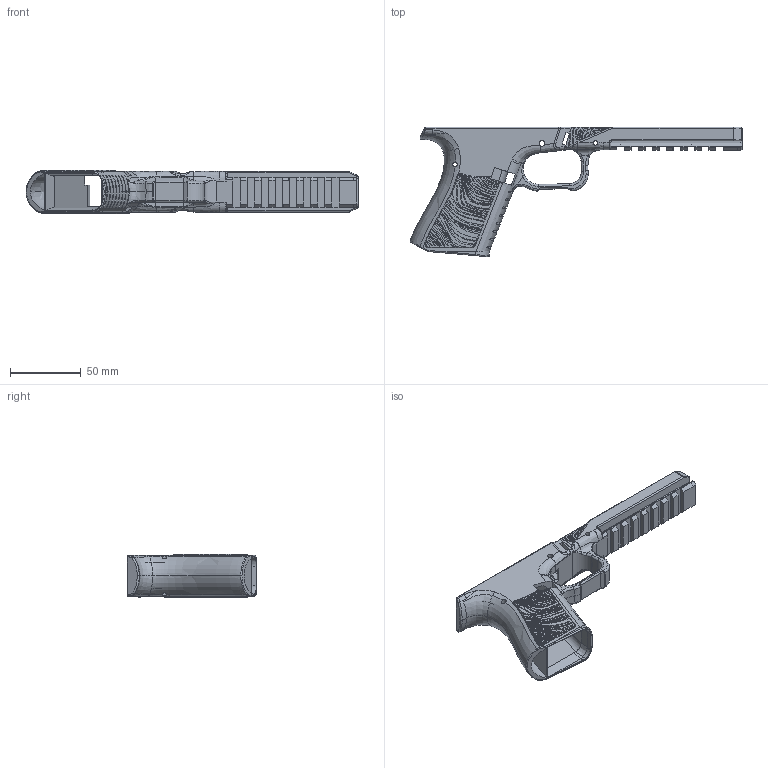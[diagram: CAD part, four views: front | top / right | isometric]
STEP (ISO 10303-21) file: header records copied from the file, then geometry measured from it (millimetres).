
FILE_DESCRIPTION(/* description */ (''),/* implementation_level */ '2;1');
FILE_NAME(/* name */ 'Railed G17LB Beskar.step',/* time_stamp */ '2021-03-15T13:43:12-06:00',/* author */ (''),/* organization */ (''),/* preprocessor_version */ 'ST-DEVELOPER v18.1',/* originating_system */ 'Autodesk Translation Framework v9.10.0.1330',/* authorisation */ '');
FILE_SCHEMA (('AUTOMOTIVE_DESIGN { 1 0 10303 214 3 1 1 }'));
Products named in the file (1): Railed Beskar LB17
Bounding box: 235.25 x 91.73 x 30.6 mm (x, y, z)
Volume: 89515.7 mm3; surface area: 54943.5 mm2
Topology: 1 solids, 1 shells, 2094 faces, 5717 edges, 3601 vertices
Faces by surface type: bspline 1160, plane 775, cylinder 137, torus 17, sphere 5
Full cylindrical faces by diameter (mm): 1.5 x2, 3.225 x2, 3.25 x2, 4.05 x2
Entity records: 104381 total; most frequent: CARTESIAN_POINT 62624, ORIENTED_EDGE 11410, EDGE_CURVE 5705, DIRECTION 5447, VERTEX_POINT 3601, LINE 2791, VECTOR 2791, EDGE_LOOP 2110
